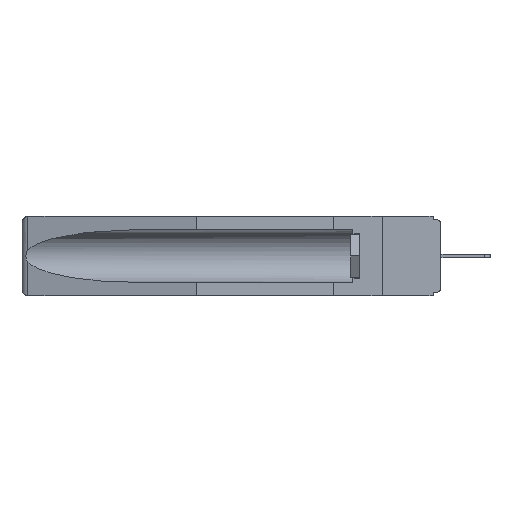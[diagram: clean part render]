
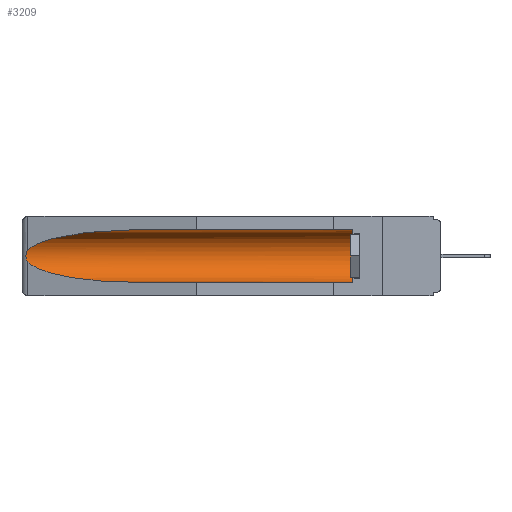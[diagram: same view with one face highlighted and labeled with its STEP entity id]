
A CAD part, left-side view. The second image highlights one B-rep face of the part: STEP entity #3209.
In plain terms, the highlighted cylindrical face has radius 2.857 mm (diameter 5.715 mm), a partial arc.
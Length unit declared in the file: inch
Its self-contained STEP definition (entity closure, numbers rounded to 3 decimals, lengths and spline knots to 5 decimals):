
#292 =( BOUNDED_CURVE ( )  B_SPLINE_CURVE ( 3, ( #10032, #7860, #977, #1416 ),
 .UNSPECIFIED., .F., .F. ) 
 B_SPLINE_CURVE_WITH_KNOTS ( ( 4, 4 ),
 ( 4.71239, 6.08839 ),
 .UNSPECIFIED. ) 
 CURVE ( )  GEOMETRIC_REPRESENTATION_ITEM ( )  RATIONAL_B_SPLINE_CURVE ( ( 1., 0.848, 0.848, 1. ) ) 
 REPRESENTATION_ITEM ( '' )  );
#360 = CYLINDRICAL_SURFACE ( 'NONE', #12698, 0.1125 ) ;
#892 = DIRECTION ( 'NONE',  ( 0., 1., 0. ) ) ;
#977 = CARTESIAN_POINT ( 'NONE',  ( 0.25451, 1.48313, -0.09465 ) ) ;
#1000 = CARTESIAN_POINT ( 'NONE',  ( 0.155, 1.07973, -0.059 ) ) ;
#1197 = CARTESIAN_POINT ( 'NONE',  ( 0.2673, 1.53269, -0.17917 ) ) ;
#1416 = CARTESIAN_POINT ( 'NONE',  ( 0.26537, 1.52718, -0.14972 ) ) ;
#1434 = CARTESIAN_POINT ( 'NONE',  ( 0.155, 0.126, -0.1715 ) ) ;
#1648 = EDGE_CURVE ( 'NONE', #8014, #6646, #292, .T. ) ;
#1690 = CARTESIAN_POINT ( 'NONE',  ( 0.21114, 1.30732, -0.284 ) ) ;
#1833 = AXIS2_PLACEMENT_3D ( 'NONE', #1434, #10478, #2743 ) ;
#2217 = CARTESIAN_POINT ( 'NONE',  ( 0.155, -0.30754, -0.284 ) ) ;
#2519 = CARTESIAN_POINT ( 'NONE',  ( 0.26597, 1.5296, -0.19026 ) ) ;
#2743 = DIRECTION ( 'NONE',  ( 0., 0., 1. ) ) ;
#3209 = ADVANCED_FACE ( 'NONE', ( #4197 ), #360, .F. ) ;
#3401 = LINE ( 'NONE', #16134, #6393 ) ;
#3542 = EDGE_CURVE ( 'NONE', #12017, #14901, #6142, .T. ) ;
#4062 = ORIENTED_EDGE ( 'NONE', *, *, #1648, .T. ) ;
#4197 = FACE_OUTER_BOUND ( 'NONE', #10131, .T. ) ;
#4386 = DIRECTION ( 'NONE',  ( 0., 1., 0. ) ) ;
#4571 = VERTEX_POINT ( 'NONE', #13749 ) ;
#5778 = CARTESIAN_POINT ( 'NONE',  ( 0.26537, 1.52718, -0.19328 ) ) ;
#6007 = EDGE_CURVE ( 'NONE', #6646, #12017, #16273, .T. ) ;
#6142 =( BOUNDED_CURVE ( )  B_SPLINE_CURVE ( 3, ( #6582, #11221, #1690, #16669 ),
 .UNSPECIFIED., .F., .F. ) 
 B_SPLINE_CURVE_WITH_KNOTS ( ( 4, 4 ),
 ( 0.1948, 1.5708 ),
 .UNSPECIFIED. ) 
 CURVE ( )  GEOMETRIC_REPRESENTATION_ITEM ( )  RATIONAL_B_SPLINE_CURVE ( ( 1., 0.848, 0.848, 1. ) ) 
 REPRESENTATION_ITEM ( '' )  );
#6393 = VECTOR ( 'NONE', #8437, 39.37008 ) ;
#6582 = CARTESIAN_POINT ( 'NONE',  ( 0.26537, 1.52718, -0.19328 ) ) ;
#6646 = VERTEX_POINT ( 'NONE', #12913 ) ;
#7391 = ORIENTED_EDGE ( 'NONE', *, *, #6007, .T. ) ;
#7517 = DIRECTION ( 'NONE',  ( 0., 0., 1. ) ) ;
#7544 = CARTESIAN_POINT ( 'NONE',  ( 0.26537, 1.52718, -0.14972 ) ) ;
#7601 = CARTESIAN_POINT ( 'NONE',  ( 0.2673, 1.5327, -0.16383 ) ) ;
#7860 = CARTESIAN_POINT ( 'NONE',  ( 0.21114, 1.30732, -0.059 ) ) ;
#8014 = VERTEX_POINT ( 'NONE', #1000 ) ;
#8152 = ORIENTED_EDGE ( 'NONE', *, *, #13040, .F. ) ;
#8437 = DIRECTION ( 'NONE',  ( 0., 1., 0. ) ) ;
#8902 = CARTESIAN_POINT ( 'NONE',  ( 0.2675, 1.53308, -0.17534 ) ) ;
#9937 = VERTEX_POINT ( 'NONE', #11741 ) ;
#10032 = CARTESIAN_POINT ( 'NONE',  ( 0.155, 1.07973, -0.059 ) ) ;
#10131 = EDGE_LOOP ( 'NONE', ( #4062, #7391, #16558, #8152, #16503, #10585 ) ) ;
#10249 = CARTESIAN_POINT ( 'NONE',  ( 0.26655, 1.53094, -0.18657 ) ) ;
#10478 = DIRECTION ( 'NONE',  ( 0., -1., 0. ) ) ;
#10585 = ORIENTED_EDGE ( 'NONE', *, *, #11399, .T. ) ;
#11221 = CARTESIAN_POINT ( 'NONE',  ( 0.25451, 1.48313, -0.24835 ) ) ;
#11399 = EDGE_CURVE ( 'NONE', #4571, #8014, #3401, .T. ) ;
#11535 = CARTESIAN_POINT ( 'NONE',  ( 0.26537, 1.52718, -0.19328 ) ) ;
#11741 = CARTESIAN_POINT ( 'NONE',  ( 0.155, 0.126, -0.284 ) ) ;
#12017 = VERTEX_POINT ( 'NONE', #5778 ) ;
#12605 = VECTOR ( 'NONE', #892, 39.37008 ) ;
#12627 = EDGE_CURVE ( 'NONE', #9937, #4571, #15211, .T. ) ;
#12698 = AXIS2_PLACEMENT_3D ( 'NONE', #16512, #4386, #7517 ) ;
#12704 = CARTESIAN_POINT ( 'NONE',  ( 0.26597, 1.52961, -0.15275 ) ) ;
#12913 = CARTESIAN_POINT ( 'NONE',  ( 0.26537, 1.52718, -0.14972 ) ) ;
#13040 = EDGE_CURVE ( 'NONE', #9937, #14901, #15980, .T. ) ;
#13749 = CARTESIAN_POINT ( 'NONE',  ( 0.155, 0.126, -0.059 ) ) ;
#14901 = VERTEX_POINT ( 'NONE', #16643 ) ;
#15211 = CIRCLE ( 'NONE', #1833, 0.1125 ) ;
#15321 = CARTESIAN_POINT ( 'NONE',  ( 0.26654, 1.53092, -0.15636 ) ) ;
#15980 = LINE ( 'NONE', #2217, #12605 ) ;
#16134 = CARTESIAN_POINT ( 'NONE',  ( 0.155, -0.30754, -0.059 ) ) ;
#16273 = B_SPLINE_CURVE_WITH_KNOTS ( 'NONE', 3,
 ( #7544, #12704, #15321, #7601, #16601, #8902, #1197, #10249, #2519, #11535 ),
 .UNSPECIFIED., .F., .F.,
 ( 4, 2, 2, 2, 4 ),
 ( 0., 0.00029, 0.00058, 0.00087, 0.00117 ),
 .UNSPECIFIED. ) ;
#16503 = ORIENTED_EDGE ( 'NONE', *, *, #12627, .T. ) ;
#16512 = CARTESIAN_POINT ( 'NONE',  ( 0.155, -0.30754, -0.1715 ) ) ;
#16558 = ORIENTED_EDGE ( 'NONE', *, *, #3542, .T. ) ;
#16601 = CARTESIAN_POINT ( 'NONE',  ( 0.2675, 1.53308, -0.16763 ) ) ;
#16643 = CARTESIAN_POINT ( 'NONE',  ( 0.155, 1.07973, -0.284 ) ) ;
#16669 = CARTESIAN_POINT ( 'NONE',  ( 0.155, 1.07973, -0.284 ) ) ;
